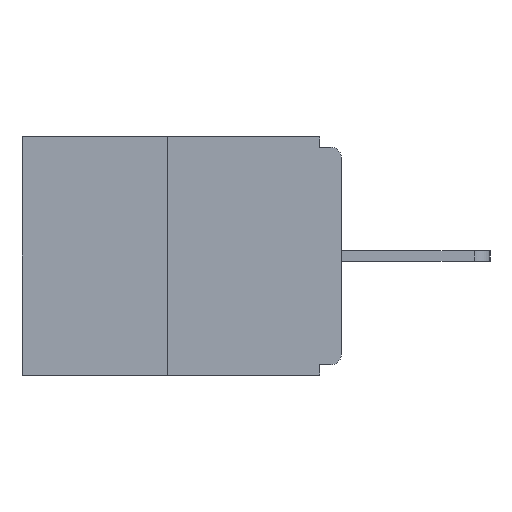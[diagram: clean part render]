
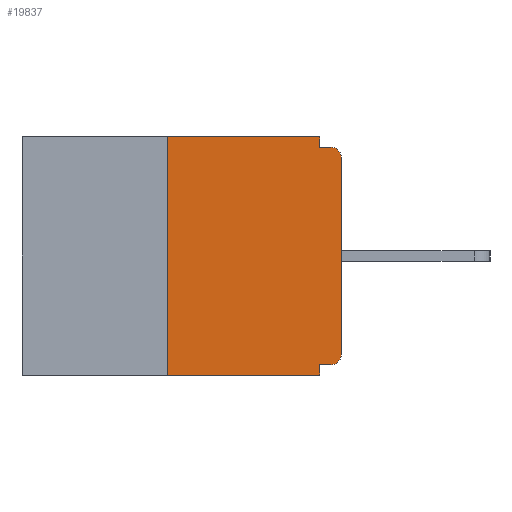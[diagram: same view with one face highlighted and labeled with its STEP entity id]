
A CAD part, left-side view. The second image highlights one B-rep face of the part: STEP entity #19837.
In plain terms, the highlighted planar face has unit normal (-1, 0, 0).
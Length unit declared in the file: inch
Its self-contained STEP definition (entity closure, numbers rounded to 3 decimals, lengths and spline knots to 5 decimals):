
#183 = CIRCLE ( 'NONE', #4082, 0.015 ) ;
#206 = DIRECTION ( 'NONE',  ( 0., -1., 0. ) ) ;
#549 = FACE_OUTER_BOUND ( 'NONE', #11017, .T. ) ;
#714 = DIRECTION ( 'NONE',  ( 0., 1., 0. ) ) ;
#811 = LINE ( 'NONE', #19277, #5602 ) ;
#1237 = CARTESIAN_POINT ( 'NONE',  ( 0., 0.015, -0.313 ) ) ;
#1576 = VERTEX_POINT ( 'NONE', #1812 ) ;
#1726 = DIRECTION ( 'NONE',  ( 0., 0., -1. ) ) ;
#1812 = CARTESIAN_POINT ( 'NONE',  ( 0., 0.015, -0.328 ) ) ;
#1881 = VERTEX_POINT ( 'NONE', #18334 ) ;
#2063 = CARTESIAN_POINT ( 'NONE',  ( 0., 0.031, -0.328 ) ) ;
#2095 = VERTEX_POINT ( 'NONE', #3859 ) ;
#2691 = CARTESIAN_POINT ( 'NONE',  ( 0., 0.015, -0.03 ) ) ;
#2701 = DIRECTION ( 'NONE',  ( 0., 0., 1. ) ) ;
#3013 = VECTOR ( 'NONE', #1726, 39.37008 ) ;
#3377 = ORIENTED_EDGE ( 'NONE', *, *, #21589, .F. ) ;
#3396 = LINE ( 'NONE', #16863, #3013 ) ;
#3859 = CARTESIAN_POINT ( 'NONE',  ( 0., 0.031, -0.015 ) ) ;
#3866 = VECTOR ( 'NONE', #6307, 39.37008 ) ;
#3882 = CARTESIAN_POINT ( 'NONE',  ( 0., 0.031, -0.343 ) ) ;
#4082 = AXIS2_PLACEMENT_3D ( 'NONE', #2691, #9384, #16147 ) ;
#4306 = EDGE_CURVE ( 'NONE', #20948, #5215, #8271, .T. ) ;
#4603 = EDGE_CURVE ( 'NONE', #8973, #15284, #12342, .T. ) ;
#4954 = EDGE_CURVE ( 'NONE', #1576, #8973, #13851, .T. ) ;
#4968 = CARTESIAN_POINT ( 'NONE',  ( 0., 0.015, -0.015 ) ) ;
#5125 = CARTESIAN_POINT ( 'NONE',  ( 0., 0., -0.03 ) ) ;
#5215 = VERTEX_POINT ( 'NONE', #6668 ) ;
#5602 = VECTOR ( 'NONE', #2701, 39.37008 ) ;
#5841 = DIRECTION ( 'NONE',  ( 0., 0., -1. ) ) ;
#6200 = DIRECTION ( 'NONE',  ( 0., 0., -1. ) ) ;
#6307 = DIRECTION ( 'NONE',  ( 0., 0., 1. ) ) ;
#6668 = CARTESIAN_POINT ( 'NONE',  ( 0., 0.25, 0. ) ) ;
#6868 = VECTOR ( 'NONE', #13410, 39.37008 ) ;
#7051 = LINE ( 'NONE', #8290, #9072 ) ;
#7263 = DIRECTION ( 'NONE',  ( 0., -1., 0. ) ) ;
#7335 = CARTESIAN_POINT ( 'NONE',  ( 0., 0., -0.328 ) ) ;
#7598 = PLANE ( 'NONE',  #20050 ) ;
#7609 = EDGE_CURVE ( 'NONE', #20948, #15284, #13287, .T. ) ;
#7630 = EDGE_CURVE ( 'NONE', #12917, #2095, #3396, .T. ) ;
#8271 = LINE ( 'NONE', #21475, #3866 ) ;
#8290 = CARTESIAN_POINT ( 'NONE',  ( 0., 0.46, 0. ) ) ;
#8973 = VERTEX_POINT ( 'NONE', #2063 ) ;
#9072 = VECTOR ( 'NONE', #7263, 39.37008 ) ;
#9149 = ORIENTED_EDGE ( 'NONE', *, *, #4603, .F. ) ;
#9384 = DIRECTION ( 'NONE',  ( -1., 0., 0. ) ) ;
#9620 = EDGE_CURVE ( 'NONE', #20978, #18410, #183, .T. ) ;
#11017 = EDGE_LOOP ( 'NONE', ( #14817, #17495, #17048, #9149, #17571, #18199, #19218, #18556, #3377, #19316 ) ) ;
#11626 = CARTESIAN_POINT ( 'NONE',  ( 0., 0.031, 0. ) ) ;
#12220 = LINE ( 'NONE', #15337, #12304 ) ;
#12226 = EDGE_CURVE ( 'NONE', #5215, #12917, #7051, .T. ) ;
#12304 = VECTOR ( 'NONE', #206, 39.37008 ) ;
#12342 = LINE ( 'NONE', #12546, #19512 ) ;
#12344 = CARTESIAN_POINT ( 'NONE',  ( 0., 0.46, 0. ) ) ;
#12546 = CARTESIAN_POINT ( 'NONE',  ( 0., 0.031, -0.343 ) ) ;
#12917 = VERTEX_POINT ( 'NONE', #11626 ) ;
#12935 = CARTESIAN_POINT ( 'NONE',  ( 0., 0.25, -0.343 ) ) ;
#13287 = LINE ( 'NONE', #18420, #6868 ) ;
#13410 = DIRECTION ( 'NONE',  ( 0., -1., 0. ) ) ;
#13851 = LINE ( 'NONE', #7335, #18023 ) ;
#14325 = DIRECTION ( 'NONE',  ( 0., 0., -1. ) ) ;
#14414 = EDGE_CURVE ( 'NONE', #1881, #20978, #811, .T. ) ;
#14817 = ORIENTED_EDGE ( 'NONE', *, *, #12226, .F. ) ;
#14905 = DIRECTION ( 'NONE',  ( -1., 0., 0. ) ) ;
#15284 = VERTEX_POINT ( 'NONE', #3882 ) ;
#15337 = CARTESIAN_POINT ( 'NONE',  ( 0., 0., -0.015 ) ) ;
#16147 = DIRECTION ( 'NONE',  ( 0., 0., -1. ) ) ;
#16863 = CARTESIAN_POINT ( 'NONE',  ( 0., 0.031, 0. ) ) ;
#17048 = ORIENTED_EDGE ( 'NONE', *, *, #7609, .T. ) ;
#17495 = ORIENTED_EDGE ( 'NONE', *, *, #4306, .F. ) ;
#17571 = ORIENTED_EDGE ( 'NONE', *, *, #4954, .F. ) ;
#17867 = EDGE_CURVE ( 'NONE', #1576, #1881, #18788, .T. ) ;
#18023 = VECTOR ( 'NONE', #714, 39.37008 ) ;
#18199 = ORIENTED_EDGE ( 'NONE', *, *, #17867, .T. ) ;
#18334 = CARTESIAN_POINT ( 'NONE',  ( 0., 0., -0.313 ) ) ;
#18410 = VERTEX_POINT ( 'NONE', #4968 ) ;
#18420 = CARTESIAN_POINT ( 'NONE',  ( 0., 0.46, -0.343 ) ) ;
#18556 = ORIENTED_EDGE ( 'NONE', *, *, #9620, .T. ) ;
#18788 = CIRCLE ( 'NONE', #20224, 0.015 ) ;
#19218 = ORIENTED_EDGE ( 'NONE', *, *, #14414, .T. ) ;
#19277 = CARTESIAN_POINT ( 'NONE',  ( 0., 0., 0. ) ) ;
#19316 = ORIENTED_EDGE ( 'NONE', *, *, #7630, .F. ) ;
#19512 = VECTOR ( 'NONE', #5841, 39.37008 ) ;
#19837 = ADVANCED_FACE ( 'NONE', ( #549 ), #7598, .F. ) ;
#20050 = AXIS2_PLACEMENT_3D ( 'NONE', #12344, #21006, #14325 ) ;
#20224 = AXIS2_PLACEMENT_3D ( 'NONE', #1237, #14905, #6200 ) ;
#20948 = VERTEX_POINT ( 'NONE', #12935 ) ;
#20978 = VERTEX_POINT ( 'NONE', #5125 ) ;
#21006 = DIRECTION ( 'NONE',  ( 1., 0., 0. ) ) ;
#21475 = CARTESIAN_POINT ( 'NONE',  ( 0., 0.25, 0. ) ) ;
#21589 = EDGE_CURVE ( 'NONE', #2095, #18410, #12220, .T. ) ;
